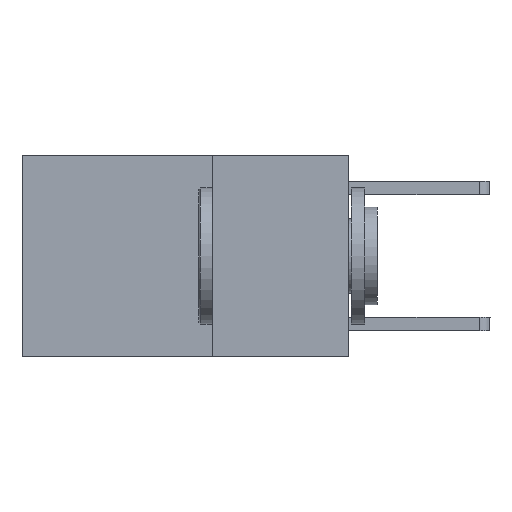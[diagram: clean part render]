
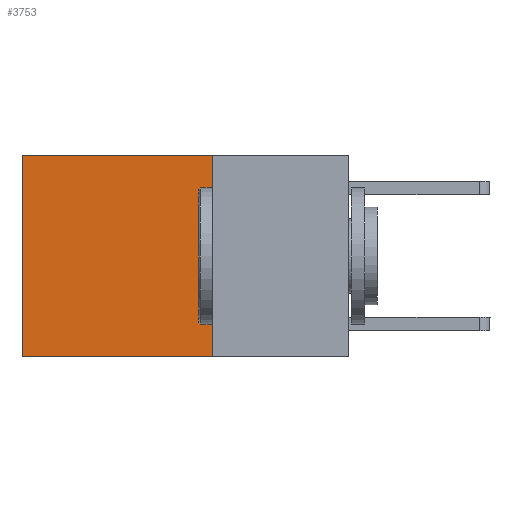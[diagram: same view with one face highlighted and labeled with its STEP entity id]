
A CAD part, left-side view. The second image highlights one B-rep face of the part: STEP entity #3753.
In plain terms, the highlighted planar face has unit normal (-1, 0, 0).
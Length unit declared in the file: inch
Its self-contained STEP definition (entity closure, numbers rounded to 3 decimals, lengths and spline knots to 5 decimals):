
#110 = CARTESIAN_POINT ( 'NONE',  ( 0.2625, 0.25, 0. ) ) ;
#179 = FACE_OUTER_BOUND ( 'NONE', #7427, .T. ) ;
#975 = EDGE_CURVE ( 'NONE', #8771, #8986, #5453, .T. ) ;
#1114 = VECTOR ( 'NONE', #7092, 39.37008 ) ;
#1701 = CARTESIAN_POINT ( 'NONE',  ( 0.2625, 0.6, -0.37 ) ) ;
#2389 = VECTOR ( 'NONE', #5381, 39.37008 ) ;
#2648 = CARTESIAN_POINT ( 'NONE',  ( 0.2625, 0.6, 0. ) ) ;
#3274 = ORIENTED_EDGE ( 'NONE', *, *, #4031, .F. ) ;
#3392 = CARTESIAN_POINT ( 'NONE',  ( 0.2625, 0.25, -0.37 ) ) ;
#3478 = AXIS2_PLACEMENT_3D ( 'NONE', #110, #3617, #7172 ) ;
#3617 = DIRECTION ( 'NONE',  ( 1., 0., 0. ) ) ;
#3633 = LINE ( 'NONE', #8904, #6197 ) ;
#3753 = ADVANCED_FACE ( 'NONE', ( #179 ), #5208, .F. ) ;
#4031 = EDGE_CURVE ( 'NONE', #8771, #8504, #5434, .T. ) ;
#4323 = ORIENTED_EDGE ( 'NONE', *, *, #6012, .T. ) ;
#5208 = PLANE ( 'NONE',  #3478 ) ;
#5381 = DIRECTION ( 'NONE',  ( 0., 0., -1. ) ) ;
#5434 = LINE ( 'NONE', #8892, #2389 ) ;
#5453 = LINE ( 'NONE', #6438, #1114 ) ;
#5483 = ORIENTED_EDGE ( 'NONE', *, *, #8221, .F. ) ;
#6012 = EDGE_CURVE ( 'NONE', #8986, #11217, #6031, .T. ) ;
#6031 = LINE ( 'NONE', #9531, #8485 ) ;
#6197 = VECTOR ( 'NONE', #10887, 39.37008 ) ;
#6438 = CARTESIAN_POINT ( 'NONE',  ( 0.2625, 0.25, 0. ) ) ;
#7092 = DIRECTION ( 'NONE',  ( 0., 1., 0. ) ) ;
#7172 = DIRECTION ( 'NONE',  ( 0., 0., -1. ) ) ;
#7427 = EDGE_LOOP ( 'NONE', ( #4323, #5483, #3274, #10702 ) ) ;
#8221 = EDGE_CURVE ( 'NONE', #8504, #11217, #3633, .T. ) ;
#8242 = CARTESIAN_POINT ( 'NONE',  ( 0.2625, 0.25, 0. ) ) ;
#8485 = VECTOR ( 'NONE', #10461, 39.37008 ) ;
#8504 = VERTEX_POINT ( 'NONE', #3392 ) ;
#8771 = VERTEX_POINT ( 'NONE', #8242 ) ;
#8892 = CARTESIAN_POINT ( 'NONE',  ( 0.2625, 0.25, 0. ) ) ;
#8904 = CARTESIAN_POINT ( 'NONE',  ( 0.2625, 0.25, -0.37 ) ) ;
#8986 = VERTEX_POINT ( 'NONE', #2648 ) ;
#9531 = CARTESIAN_POINT ( 'NONE',  ( 0.2625, 0.6, 0. ) ) ;
#10461 = DIRECTION ( 'NONE',  ( 0., 0., -1. ) ) ;
#10702 = ORIENTED_EDGE ( 'NONE', *, *, #975, .T. ) ;
#10887 = DIRECTION ( 'NONE',  ( 0., 1., 0. ) ) ;
#11217 = VERTEX_POINT ( 'NONE', #1701 ) ;
